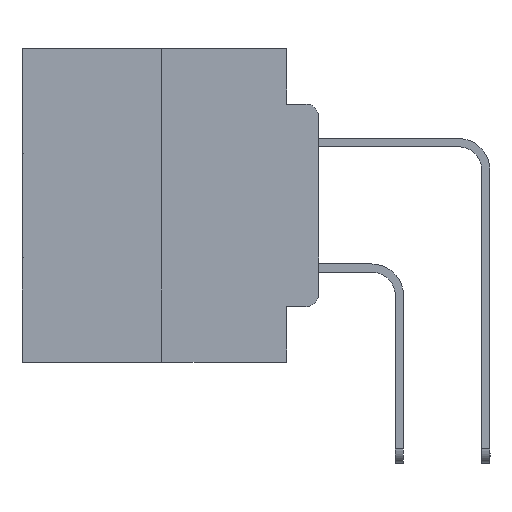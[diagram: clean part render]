
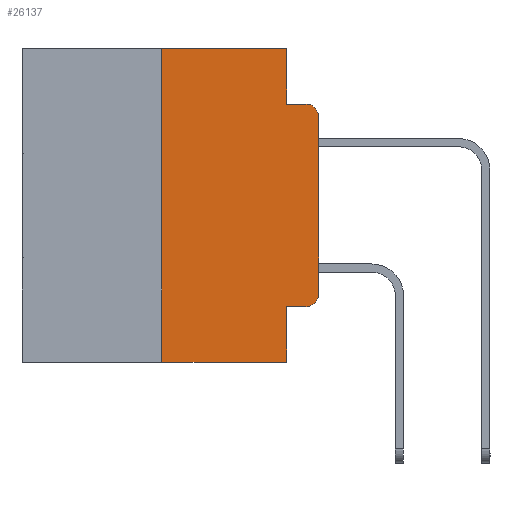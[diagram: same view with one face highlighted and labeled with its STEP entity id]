
A CAD part, left-side view. The second image highlights one B-rep face of the part: STEP entity #26137.
In plain terms, the highlighted planar face has unit normal (-1, 0, 0).
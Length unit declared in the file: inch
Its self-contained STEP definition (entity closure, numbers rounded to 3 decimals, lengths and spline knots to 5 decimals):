
#744 = ORIENTED_EDGE ( 'NONE', *, *, #3845, .F. ) ;
#952 = VERTEX_POINT ( 'NONE', #8700 ) ;
#1036 = EDGE_CURVE ( 'NONE', #5363, #14937, #14912, .T. ) ;
#1673 = EDGE_CURVE ( 'NONE', #11809, #7844, #13413, .T. ) ;
#1789 = DIRECTION ( 'NONE',  ( 0., 0., -1. ) ) ;
#1923 = LINE ( 'NONE', #25920, #29139 ) ;
#2002 = ORIENTED_EDGE ( 'NONE', *, *, #10259, .T. ) ;
#2679 = ORIENTED_EDGE ( 'NONE', *, *, #13860, .T. ) ;
#3845 = EDGE_CURVE ( 'NONE', #24304, #16726, #1923, .T. ) ;
#4627 = CARTESIAN_POINT ( 'NONE',  ( 0., 0.051, 0. ) ) ;
#4859 = VECTOR ( 'NONE', #19299, 39.37008 ) ;
#5303 = ORIENTED_EDGE ( 'NONE', *, *, #23990, .F. ) ;
#5363 = VERTEX_POINT ( 'NONE', #5985 ) ;
#5549 = CARTESIAN_POINT ( 'NONE',  ( 0., 0.051, 0. ) ) ;
#5754 = AXIS2_PLACEMENT_3D ( 'NONE', #25055, #27326, #6938 ) ;
#5985 = CARTESIAN_POINT ( 'NONE',  ( 0., 0.02, -0.4115 ) ) ;
#6103 = CARTESIAN_POINT ( 'NONE',  ( 0., 0.473, 0. ) ) ;
#6938 = DIRECTION ( 'NONE',  ( 0., 0., -1. ) ) ;
#6957 = VERTEX_POINT ( 'NONE', #5549 ) ;
#7370 = VECTOR ( 'NONE', #1789, 39.37008 ) ;
#7844 = VERTEX_POINT ( 'NONE', #21872 ) ;
#8700 = CARTESIAN_POINT ( 'NONE',  ( 0., 0.25, 0. ) ) ;
#8764 = CARTESIAN_POINT ( 'NONE',  ( 0., 0.02, -0.0885 ) ) ;
#9957 = CARTESIAN_POINT ( 'NONE',  ( 0., 0., -0.3915 ) ) ;
#9990 = LINE ( 'NONE', #19901, #19243 ) ;
#10059 = EDGE_LOOP ( 'NONE', ( #2002, #25167, #744, #27322, #5303, #10221, #18789, #17738, #2679, #25264 ) ) ;
#10221 = ORIENTED_EDGE ( 'NONE', *, *, #19686, .F. ) ;
#10259 = EDGE_CURVE ( 'NONE', #14937, #18227, #19648, .T. ) ;
#10554 = CIRCLE ( 'NONE', #16382, 0.02 ) ;
#11026 = LINE ( 'NONE', #20171, #18155 ) ;
#11809 = VERTEX_POINT ( 'NONE', #26792 ) ;
#12167 = DIRECTION ( 'NONE',  ( 0., -1., 0. ) ) ;
#12576 = DIRECTION ( 'NONE',  ( -1., 0., 0. ) ) ;
#13413 = LINE ( 'NONE', #13568, #7370 ) ;
#13568 = CARTESIAN_POINT ( 'NONE',  ( 0., 0.051, 0. ) ) ;
#13860 = EDGE_CURVE ( 'NONE', #11809, #5363, #26616, .T. ) ;
#14469 = DIRECTION ( 'NONE',  ( 0., 0., -1. ) ) ;
#14679 = FACE_OUTER_BOUND ( 'NONE', #10059, .T. ) ;
#14696 = VECTOR ( 'NONE', #20054, 39.37008 ) ;
#14912 = CIRCLE ( 'NONE', #5754, 0.02 ) ;
#14937 = VERTEX_POINT ( 'NONE', #9957 ) ;
#15237 = DIRECTION ( 'NONE',  ( 0., 0., -1. ) ) ;
#15435 = EDGE_CURVE ( 'NONE', #18227, #16726, #10554, .T. ) ;
#15511 = CARTESIAN_POINT ( 'NONE',  ( 0., 0., 0. ) ) ;
#16382 = AXIS2_PLACEMENT_3D ( 'NONE', #21317, #12576, #14469 ) ;
#16488 = EDGE_CURVE ( 'NONE', #6957, #24304, #23271, .T. ) ;
#16726 = VERTEX_POINT ( 'NONE', #8764 ) ;
#16880 = CARTESIAN_POINT ( 'NONE',  ( 0., 0.25, -0.5 ) ) ;
#17738 = ORIENTED_EDGE ( 'NONE', *, *, #1673, .F. ) ;
#17906 = DIRECTION ( 'NONE',  ( 0., -1., 0. ) ) ;
#18155 = VECTOR ( 'NONE', #24789, 39.37008 ) ;
#18227 = VERTEX_POINT ( 'NONE', #24420 ) ;
#18789 = ORIENTED_EDGE ( 'NONE', *, *, #23848, .T. ) ;
#19243 = VECTOR ( 'NONE', #24700, 39.37008 ) ;
#19299 = DIRECTION ( 'NONE',  ( 0., 0., 1. ) ) ;
#19597 = VECTOR ( 'NONE', #17906, 39.37008 ) ;
#19648 = LINE ( 'NONE', #15511, #14696 ) ;
#19686 = EDGE_CURVE ( 'NONE', #27252, #952, #25058, .T. ) ;
#19765 = VECTOR ( 'NONE', #20495, 39.37008 ) ;
#19901 = CARTESIAN_POINT ( 'NONE',  ( 0., 0.473, -0.5 ) ) ;
#20054 = DIRECTION ( 'NONE',  ( 0., 0., 1. ) ) ;
#20171 = CARTESIAN_POINT ( 'NONE',  ( 0., 0.473, 0. ) ) ;
#20495 = DIRECTION ( 'NONE',  ( 0., 0., -1. ) ) ;
#21317 = CARTESIAN_POINT ( 'NONE',  ( 0., 0.02, -0.1085 ) ) ;
#21372 = CARTESIAN_POINT ( 'NONE',  ( 0., 0.25, 0. ) ) ;
#21872 = CARTESIAN_POINT ( 'NONE',  ( 0., 0.051, -0.5 ) ) ;
#23271 = LINE ( 'NONE', #4627, #19765 ) ;
#23835 = PLANE ( 'NONE',  #26377 ) ;
#23848 = EDGE_CURVE ( 'NONE', #27252, #7844, #9990, .T. ) ;
#23990 = EDGE_CURVE ( 'NONE', #952, #6957, #11026, .T. ) ;
#24304 = VERTEX_POINT ( 'NONE', #28040 ) ;
#24420 = CARTESIAN_POINT ( 'NONE',  ( 0., 0., -0.1085 ) ) ;
#24693 = CARTESIAN_POINT ( 'NONE',  ( 0., 0.051, -0.4115 ) ) ;
#24700 = DIRECTION ( 'NONE',  ( 0., -1., 0. ) ) ;
#24789 = DIRECTION ( 'NONE',  ( 0., -1., 0. ) ) ;
#25055 = CARTESIAN_POINT ( 'NONE',  ( 0., 0.02, -0.3915 ) ) ;
#25058 = LINE ( 'NONE', #21372, #4859 ) ;
#25167 = ORIENTED_EDGE ( 'NONE', *, *, #15435, .T. ) ;
#25264 = ORIENTED_EDGE ( 'NONE', *, *, #1036, .T. ) ;
#25920 = CARTESIAN_POINT ( 'NONE',  ( 0., 0.051, -0.0885 ) ) ;
#26137 = ADVANCED_FACE ( 'NONE', ( #14679 ), #23835, .F. ) ;
#26377 = AXIS2_PLACEMENT_3D ( 'NONE', #6103, #26386, #15237 ) ;
#26386 = DIRECTION ( 'NONE',  ( 1., 0., 0. ) ) ;
#26616 = LINE ( 'NONE', #24693, #19597 ) ;
#26792 = CARTESIAN_POINT ( 'NONE',  ( 0., 0.051, -0.4115 ) ) ;
#27252 = VERTEX_POINT ( 'NONE', #16880 ) ;
#27322 = ORIENTED_EDGE ( 'NONE', *, *, #16488, .F. ) ;
#27326 = DIRECTION ( 'NONE',  ( -1., 0., 0. ) ) ;
#28040 = CARTESIAN_POINT ( 'NONE',  ( 0., 0.051, -0.0885 ) ) ;
#29139 = VECTOR ( 'NONE', #12167, 39.37008 ) ;
